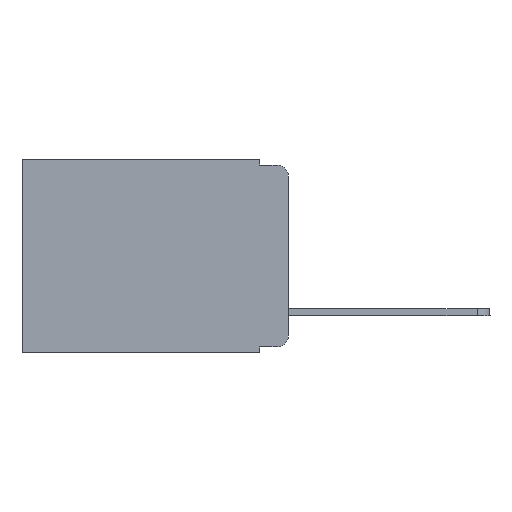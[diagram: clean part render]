
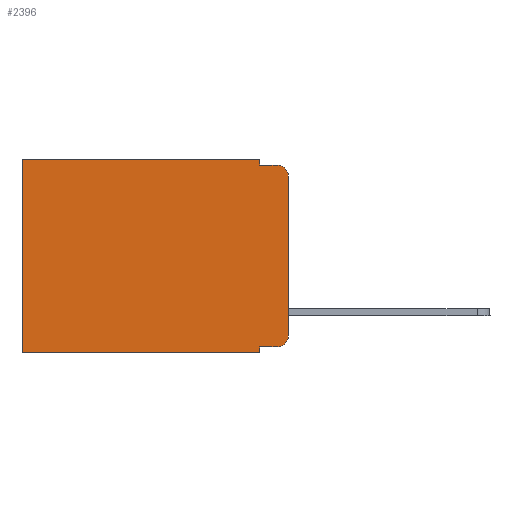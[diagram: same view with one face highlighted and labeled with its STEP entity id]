
A CAD part, left-side view. The second image highlights one B-rep face of the part: STEP entity #2396.
In plain terms, the highlighted planar face has unit normal (-1, 0, 0).
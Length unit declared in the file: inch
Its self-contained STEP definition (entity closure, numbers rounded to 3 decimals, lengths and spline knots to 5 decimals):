
#360 = DIRECTION ( 'NONE',  ( 0., 1., 0. ) ) ;
#707 = EDGE_CURVE ( 'NONE', #834, #18324, #6786, .T. ) ;
#834 = VERTEX_POINT ( 'NONE', #19347 ) ;
#1104 = EDGE_CURVE ( 'NONE', #7679, #8461, #17340, .T. ) ;
#1891 = LINE ( 'NONE', #10110, #3359 ) ;
#2014 = ORIENTED_EDGE ( 'NONE', *, *, #1104, .F. ) ;
#2216 = DIRECTION ( 'NONE',  ( 0., -1., 0. ) ) ;
#2396 = ADVANCED_FACE ( 'NONE', ( #8016 ), #15583, .F. ) ;
#2581 = LINE ( 'NONE', #5416, #9410 ) ;
#2603 = CARTESIAN_POINT ( 'NONE',  ( 0.298, 0., -0.313 ) ) ;
#2652 = AXIS2_PLACEMENT_3D ( 'NONE', #8012, #8282, #13113 ) ;
#2854 = VECTOR ( 'NONE', #18833, 39.37008 ) ;
#3091 = VECTOR ( 'NONE', #8407, 39.37008 ) ;
#3192 = VECTOR ( 'NONE', #15104, 39.37008 ) ;
#3359 = VECTOR ( 'NONE', #10175, 39.37008 ) ;
#3669 = VERTEX_POINT ( 'NONE', #9798 ) ;
#3796 = VECTOR ( 'NONE', #17806, 39.37008 ) ;
#4268 = ORIENTED_EDGE ( 'NONE', *, *, #707, .T. ) ;
#4827 = ORIENTED_EDGE ( 'NONE', *, *, #16759, .T. ) ;
#4898 = CARTESIAN_POINT ( 'NONE',  ( 0.298, 0., 0. ) ) ;
#5031 = VERTEX_POINT ( 'NONE', #8451 ) ;
#5077 = VECTOR ( 'NONE', #360, 39.37008 ) ;
#5416 = CARTESIAN_POINT ( 'NONE',  ( 0.298, 0.051, -0.333 ) ) ;
#6061 = ORIENTED_EDGE ( 'NONE', *, *, #16440, .T. ) ;
#6719 = AXIS2_PLACEMENT_3D ( 'NONE', #12042, #13659, #11969 ) ;
#6786 = LINE ( 'NONE', #14203, #5077 ) ;
#6995 = VERTEX_POINT ( 'NONE', #19891 ) ;
#7062 = AXIS2_PLACEMENT_3D ( 'NONE', #4898, #11397, #15039 ) ;
#7268 = LINE ( 'NONE', #11742, #3091 ) ;
#7447 = ORIENTED_EDGE ( 'NONE', *, *, #9346, .T. ) ;
#7679 = VERTEX_POINT ( 'NONE', #18112 ) ;
#7850 = CARTESIAN_POINT ( 'NONE',  ( 0.298, 0.051, -0.01 ) ) ;
#8012 = CARTESIAN_POINT ( 'NONE',  ( 0.298, 0.02, -0.313 ) ) ;
#8016 = FACE_OUTER_BOUND ( 'NONE', #11829, .T. ) ;
#8282 = DIRECTION ( 'NONE',  ( -1., 0., 0. ) ) ;
#8407 = DIRECTION ( 'NONE',  ( 0., 0., -1. ) ) ;
#8451 = CARTESIAN_POINT ( 'NONE',  ( 0.298, 0., -0.03 ) ) ;
#8461 = VERTEX_POINT ( 'NONE', #17972 ) ;
#8590 = VERTEX_POINT ( 'NONE', #20026 ) ;
#8711 = ORIENTED_EDGE ( 'NONE', *, *, #15146, .F. ) ;
#8954 = CARTESIAN_POINT ( 'NONE',  ( 0.298, 0.473, 0. ) ) ;
#9229 = VECTOR ( 'NONE', #19759, 39.37008 ) ;
#9305 = VERTEX_POINT ( 'NONE', #18245 ) ;
#9346 = EDGE_CURVE ( 'NONE', #18324, #6995, #16956, .T. ) ;
#9410 = VECTOR ( 'NONE', #2216, 39.37008 ) ;
#9798 = CARTESIAN_POINT ( 'NONE',  ( 0.298, 0.051, -0.333 ) ) ;
#9846 = ORIENTED_EDGE ( 'NONE', *, *, #16337, .T. ) ;
#10110 = CARTESIAN_POINT ( 'NONE',  ( 0.298, 0.051, 0. ) ) ;
#10175 = DIRECTION ( 'NONE',  ( 0., 0., -1. ) ) ;
#11397 = DIRECTION ( 'NONE',  ( 1., 0., 0. ) ) ;
#11496 = ORIENTED_EDGE ( 'NONE', *, *, #12757, .F. ) ;
#11742 = CARTESIAN_POINT ( 'NONE',  ( 0.298, 0., 0. ) ) ;
#11829 = EDGE_LOOP ( 'NONE', ( #11496, #4827, #2014, #8711, #4268, #7447, #14357, #11962, #9846, #6061 ) ) ;
#11857 = CIRCLE ( 'NONE', #6719, 0.02 ) ;
#11930 = VERTEX_POINT ( 'NONE', #2603 ) ;
#11962 = ORIENTED_EDGE ( 'NONE', *, *, #15408, .F. ) ;
#11969 = DIRECTION ( 'NONE',  ( 0., 0., -1. ) ) ;
#12042 = CARTESIAN_POINT ( 'NONE',  ( 0.298, 0.02, -0.03 ) ) ;
#12638 = LINE ( 'NONE', #14973, #9229 ) ;
#12757 = EDGE_CURVE ( 'NONE', #5031, #11930, #7268, .T. ) ;
#12893 = CARTESIAN_POINT ( 'NONE',  ( 0.298, 0., -0.343 ) ) ;
#13113 = DIRECTION ( 'NONE',  ( 0., 0., -1. ) ) ;
#13659 = DIRECTION ( 'NONE',  ( -1., 0., 0. ) ) ;
#13674 = CARTESIAN_POINT ( 'NONE',  ( 0.298, 0.473, 0. ) ) ;
#14203 = CARTESIAN_POINT ( 'NONE',  ( 0.298, 0., 0. ) ) ;
#14357 = ORIENTED_EDGE ( 'NONE', *, *, #17526, .F. ) ;
#14795 = CIRCLE ( 'NONE', #2652, 0.02 ) ;
#14973 = CARTESIAN_POINT ( 'NONE',  ( 0.298, 0.051, 0. ) ) ;
#15039 = DIRECTION ( 'NONE',  ( 0., 0., -1. ) ) ;
#15104 = DIRECTION ( 'NONE',  ( 0., 0., -1. ) ) ;
#15146 = EDGE_CURVE ( 'NONE', #834, #7679, #1891, .T. ) ;
#15408 = EDGE_CURVE ( 'NONE', #3669, #8590, #12638, .T. ) ;
#15540 = LINE ( 'NONE', #12893, #3796 ) ;
#15583 = PLANE ( 'NONE',  #7062 ) ;
#16337 = EDGE_CURVE ( 'NONE', #3669, #9305, #2581, .T. ) ;
#16440 = EDGE_CURVE ( 'NONE', #9305, #11930, #14795, .T. ) ;
#16759 = EDGE_CURVE ( 'NONE', #5031, #8461, #11857, .T. ) ;
#16956 = LINE ( 'NONE', #8954, #3192 ) ;
#17340 = LINE ( 'NONE', #7850, #2854 ) ;
#17526 = EDGE_CURVE ( 'NONE', #8590, #6995, #15540, .T. ) ;
#17806 = DIRECTION ( 'NONE',  ( 0., 1., 0. ) ) ;
#17972 = CARTESIAN_POINT ( 'NONE',  ( 0.298, 0.02, -0.01 ) ) ;
#18112 = CARTESIAN_POINT ( 'NONE',  ( 0.298, 0.051, -0.01 ) ) ;
#18245 = CARTESIAN_POINT ( 'NONE',  ( 0.298, 0.02, -0.333 ) ) ;
#18324 = VERTEX_POINT ( 'NONE', #13674 ) ;
#18833 = DIRECTION ( 'NONE',  ( 0., -1., 0. ) ) ;
#19347 = CARTESIAN_POINT ( 'NONE',  ( 0.298, 0.051, 0. ) ) ;
#19759 = DIRECTION ( 'NONE',  ( 0., 0., -1. ) ) ;
#19891 = CARTESIAN_POINT ( 'NONE',  ( 0.298, 0.473, -0.343 ) ) ;
#20026 = CARTESIAN_POINT ( 'NONE',  ( 0.298, 0.051, -0.343 ) ) ;
